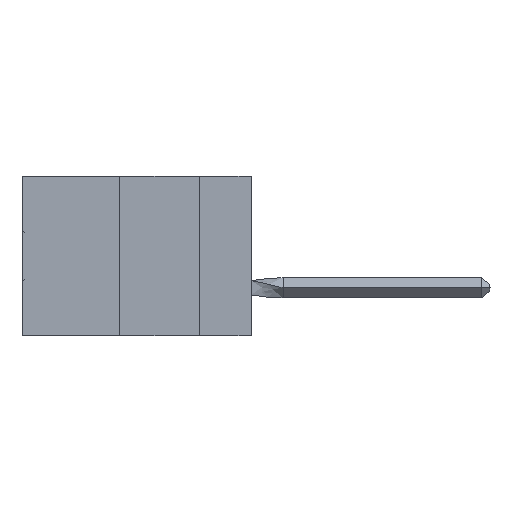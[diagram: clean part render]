
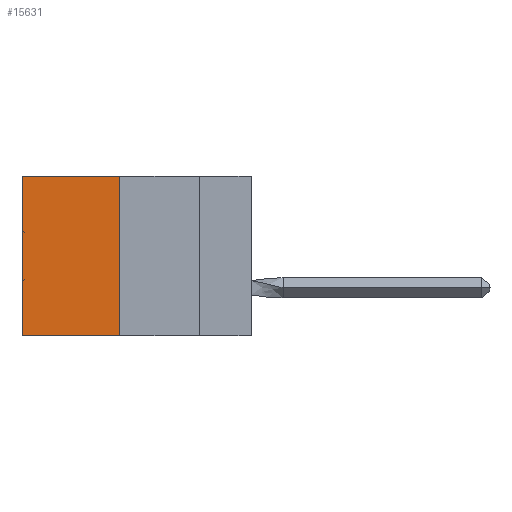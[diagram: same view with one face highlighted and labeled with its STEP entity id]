
A CAD part, left-side view. The second image highlights one B-rep face of the part: STEP entity #15631.
In plain terms, the highlighted planar face has unit normal (-1, 0, 0).
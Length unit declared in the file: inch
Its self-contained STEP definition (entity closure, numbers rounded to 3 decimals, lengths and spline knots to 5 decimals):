
#1524 = CARTESIAN_POINT ( 'NONE',  ( 0.305, 0.72, -0.5 ) ) ;
#4635 = VECTOR ( 'NONE', #10850, 39.37008 ) ;
#6424 = CARTESIAN_POINT ( 'NONE',  ( 0.305, 0.413, -0.5 ) ) ;
#7415 = CARTESIAN_POINT ( 'NONE',  ( 0.305, 0.413, -0.5 ) ) ;
#8712 = FACE_OUTER_BOUND ( 'NONE', #45725, .T. ) ;
#8735 = AXIS2_PLACEMENT_3D ( 'NONE', #6424, #18690, #22525 ) ;
#9054 = LINE ( 'NONE', #12179, #47867 ) ;
#10439 = ORIENTED_EDGE ( 'NONE', *, *, #13165, .F. ) ;
#10850 = DIRECTION ( 'NONE',  ( 0., 1., 0. ) ) ;
#12023 = EDGE_CURVE ( 'NONE', #37653, #39617, #9054, .T. ) ;
#12179 = CARTESIAN_POINT ( 'NONE',  ( 0.305, 0.413, -0.5 ) ) ;
#13165 = EDGE_CURVE ( 'NONE', #41991, #37653, #30234, .T. ) ;
#13632 = DIRECTION ( 'NONE',  ( 0., 0., -1. ) ) ;
#14033 = VECTOR ( 'NONE', #13632, 39.37008 ) ;
#15631 = ADVANCED_FACE ( 'NONE', ( #8712 ), #42671, .F. ) ;
#15896 = LINE ( 'NONE', #22893, #4635 ) ;
#16094 = CARTESIAN_POINT ( 'NONE',  ( 0.305, 0.72, 0. ) ) ;
#18690 = DIRECTION ( 'NONE',  ( 1., 0., 0. ) ) ;
#19598 = VECTOR ( 'NONE', #47333, 39.37008 ) ;
#22478 = EDGE_CURVE ( 'NONE', #41991, #43734, #15896, .T. ) ;
#22525 = DIRECTION ( 'NONE',  ( 0., 0., -1. ) ) ;
#22893 = CARTESIAN_POINT ( 'NONE',  ( 0.305, 0.413, 0. ) ) ;
#22931 = ORIENTED_EDGE ( 'NONE', *, *, #30984, .T. ) ;
#24656 = LINE ( 'NONE', #49507, #14033 ) ;
#25108 = CARTESIAN_POINT ( 'NONE',  ( 0.305, 0.413, -0.5 ) ) ;
#27532 = ORIENTED_EDGE ( 'NONE', *, *, #22478, .T. ) ;
#28461 = DIRECTION ( 'NONE',  ( 0., 1., 0. ) ) ;
#30234 = LINE ( 'NONE', #7415, #19598 ) ;
#30984 = EDGE_CURVE ( 'NONE', #43734, #39617, #24656, .T. ) ;
#36333 = CARTESIAN_POINT ( 'NONE',  ( 0.305, 0.413, 0. ) ) ;
#37653 = VERTEX_POINT ( 'NONE', #25108 ) ;
#39617 = VERTEX_POINT ( 'NONE', #1524 ) ;
#41942 = ORIENTED_EDGE ( 'NONE', *, *, #12023, .F. ) ;
#41991 = VERTEX_POINT ( 'NONE', #36333 ) ;
#42671 = PLANE ( 'NONE',  #8735 ) ;
#43734 = VERTEX_POINT ( 'NONE', #16094 ) ;
#45725 = EDGE_LOOP ( 'NONE', ( #22931, #41942, #10439, #27532 ) ) ;
#47333 = DIRECTION ( 'NONE',  ( 0., 0., -1. ) ) ;
#47867 = VECTOR ( 'NONE', #28461, 39.37008 ) ;
#49507 = CARTESIAN_POINT ( 'NONE',  ( 0.305, 0.72, -0.5 ) ) ;
